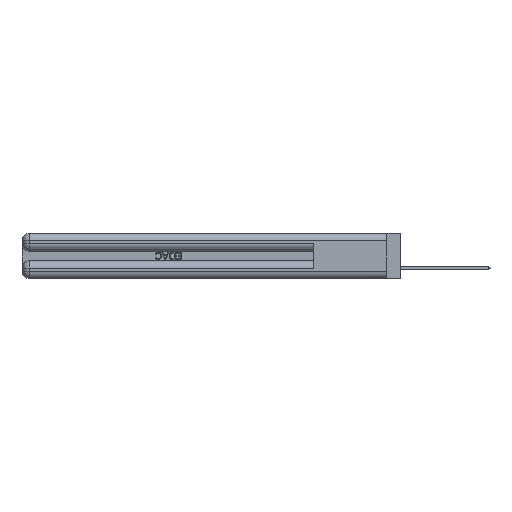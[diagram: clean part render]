
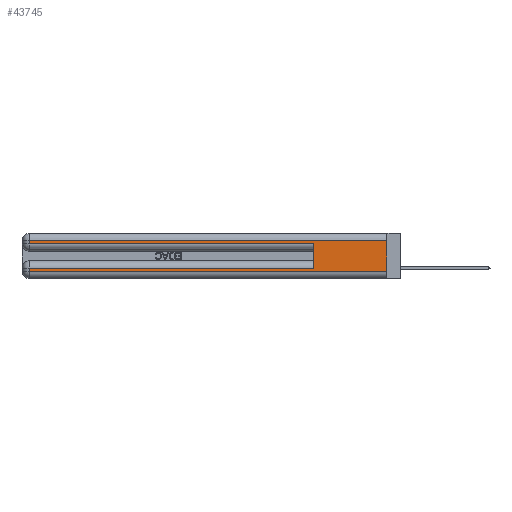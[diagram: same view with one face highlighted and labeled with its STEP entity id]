
A CAD part, left-side view. The second image highlights one B-rep face of the part: STEP entity #43745.
In plain terms, the highlighted planar face has unit normal (-1, 0, 0).
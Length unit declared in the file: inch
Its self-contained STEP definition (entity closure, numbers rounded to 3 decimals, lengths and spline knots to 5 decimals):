
#815 = CARTESIAN_POINT ( 'NONE',  ( 0., 2.94, 0.37 ) ) ;
#1247 = CARTESIAN_POINT ( 'NONE',  ( 0., 0.6, 0.285 ) ) ;
#1469 = VECTOR ( 'NONE', #23789, 39.37008 ) ;
#1669 = VERTEX_POINT ( 'NONE', #33736 ) ;
#1790 = CARTESIAN_POINT ( 'NONE',  ( 0., 0., 0.06 ) ) ;
#2220 = FACE_OUTER_BOUND ( 'NONE', #28199, .T. ) ;
#2231 = EDGE_CURVE ( 'NONE', #16313, #1669, #24811, .T. ) ;
#2413 = LINE ( 'NONE', #40685, #35208 ) ;
#5345 = VERTEX_POINT ( 'NONE', #1790 ) ;
#7798 = CARTESIAN_POINT ( 'NONE',  ( 0., 0., 0.31 ) ) ;
#8728 = ORIENTED_EDGE ( 'NONE', *, *, #20245, .T. ) ;
#13500 = VECTOR ( 'NONE', #22282, 39.37008 ) ;
#14312 = CARTESIAN_POINT ( 'NONE',  ( 0., 0., 0.085 ) ) ;
#14416 = ORIENTED_EDGE ( 'NONE', *, *, #2231, .T. ) ;
#15192 = VERTEX_POINT ( 'NONE', #28647 ) ;
#16313 = VERTEX_POINT ( 'NONE', #7798 ) ;
#17002 = CARTESIAN_POINT ( 'NONE',  ( 0., 0., 0.37 ) ) ;
#17530 = LINE ( 'NONE', #23030, #44447 ) ;
#17873 = EDGE_CURVE ( 'NONE', #39191, #54982, #2413, .T. ) ;
#19131 = DIRECTION ( 'NONE',  ( 0., 0., -1. ) ) ;
#20245 = EDGE_CURVE ( 'NONE', #15192, #31103, #42331, .T. ) ;
#20575 = ORIENTED_EDGE ( 'NONE', *, *, #44324, .F. ) ;
#21261 = VECTOR ( 'NONE', #31246, 39.37008 ) ;
#21999 = EDGE_CURVE ( 'NONE', #54982, #5345, #55481, .T. ) ;
#22282 = DIRECTION ( 'NONE',  ( 0., 0., -1. ) ) ;
#22939 = DIRECTION ( 'NONE',  ( 0., 1., 0. ) ) ;
#23030 = CARTESIAN_POINT ( 'NONE',  ( 0., 0.6, 0.145 ) ) ;
#23789 = DIRECTION ( 'NONE',  ( 0., -1., 0. ) ) ;
#24668 = DIRECTION ( 'NONE',  ( 0., 1., 0. ) ) ;
#24811 = LINE ( 'NONE', #40611, #48973 ) ;
#26636 = VERTEX_POINT ( 'NONE', #35037 ) ;
#27306 = DIRECTION ( 'NONE',  ( 0., 0., 1. ) ) ;
#28053 = CARTESIAN_POINT ( 'NONE',  ( 0., 0., 0.285 ) ) ;
#28199 = EDGE_LOOP ( 'NONE', ( #33424, #14416, #31900, #8728, #20575, #54021, #32356, #37341 ) ) ;
#28647 = CARTESIAN_POINT ( 'NONE',  ( 0., 2.94, 0.285 ) ) ;
#28973 = PLANE ( 'NONE',  #41937 ) ;
#29356 = CARTESIAN_POINT ( 'NONE',  ( 0., 0., 0.37 ) ) ;
#30223 = CARTESIAN_POINT ( 'NONE',  ( 0., 2.94, 0.085 ) ) ;
#31103 = VERTEX_POINT ( 'NONE', #1247 ) ;
#31246 = DIRECTION ( 'NONE',  ( 0., -1., 0. ) ) ;
#31900 = ORIENTED_EDGE ( 'NONE', *, *, #44199, .T. ) ;
#32356 = ORIENTED_EDGE ( 'NONE', *, *, #17873, .T. ) ;
#33424 = ORIENTED_EDGE ( 'NONE', *, *, #40331, .F. ) ;
#33736 = CARTESIAN_POINT ( 'NONE',  ( 0., 2.94, 0.31 ) ) ;
#33995 = EDGE_CURVE ( 'NONE', #26636, #39191, #41193, .T. ) ;
#35037 = CARTESIAN_POINT ( 'NONE',  ( 0., 0.6, 0.085 ) ) ;
#35208 = VECTOR ( 'NONE', #19131, 39.37008 ) ;
#35341 = DIRECTION ( 'NONE',  ( 0., 0., -1. ) ) ;
#37341 = ORIENTED_EDGE ( 'NONE', *, *, #21999, .T. ) ;
#39191 = VERTEX_POINT ( 'NONE', #30223 ) ;
#40331 = EDGE_CURVE ( 'NONE', #16313, #5345, #42819, .T. ) ;
#40402 = LINE ( 'NONE', #815, #13500 ) ;
#40522 = DIRECTION ( 'NONE',  ( 1., 0., 0. ) ) ;
#40611 = CARTESIAN_POINT ( 'NONE',  ( 0., 0., 0.31 ) ) ;
#40685 = CARTESIAN_POINT ( 'NONE',  ( 0., 2.94, 0.37 ) ) ;
#41193 = LINE ( 'NONE', #14312, #47921 ) ;
#41937 = AXIS2_PLACEMENT_3D ( 'NONE', #17002, #40522, #35341 ) ;
#42331 = LINE ( 'NONE', #28053, #1469 ) ;
#42502 = DIRECTION ( 'NONE',  ( 0., 0., -1. ) ) ;
#42819 = LINE ( 'NONE', #29356, #52223 ) ;
#43745 = ADVANCED_FACE ( 'NONE', ( #2220 ), #28973, .F. ) ;
#44033 = CARTESIAN_POINT ( 'NONE',  ( 0., 0., 0.06 ) ) ;
#44199 = EDGE_CURVE ( 'NONE', #1669, #15192, #40402, .T. ) ;
#44324 = EDGE_CURVE ( 'NONE', #26636, #31103, #17530, .T. ) ;
#44447 = VECTOR ( 'NONE', #27306, 39.37008 ) ;
#47921 = VECTOR ( 'NONE', #22939, 39.37008 ) ;
#48973 = VECTOR ( 'NONE', #24668, 39.37008 ) ;
#52223 = VECTOR ( 'NONE', #42502, 39.37008 ) ;
#53958 = CARTESIAN_POINT ( 'NONE',  ( 0., 2.94, 0.06 ) ) ;
#54021 = ORIENTED_EDGE ( 'NONE', *, *, #33995, .T. ) ;
#54982 = VERTEX_POINT ( 'NONE', #53958 ) ;
#55481 = LINE ( 'NONE', #44033, #21261 ) ;
